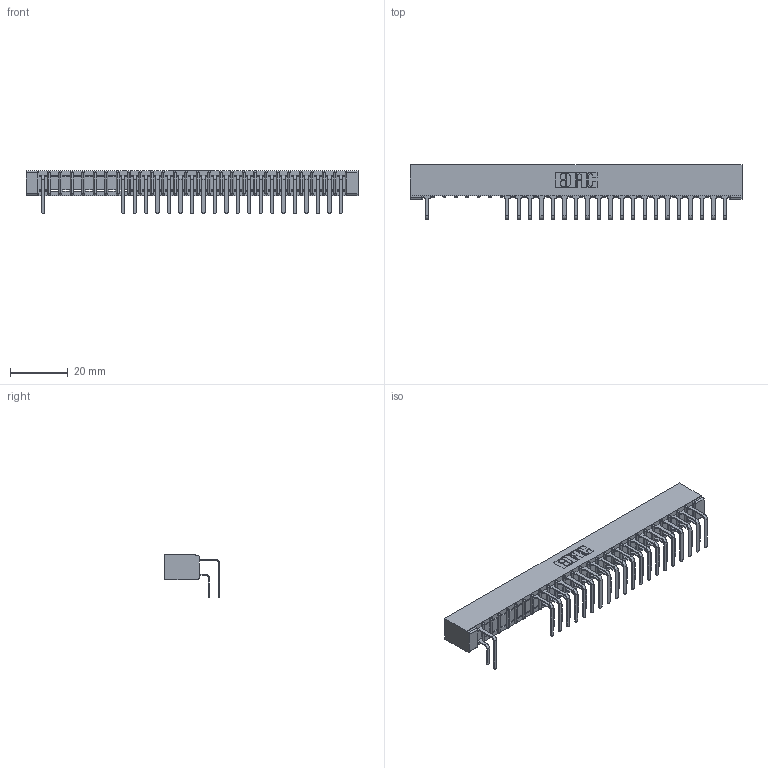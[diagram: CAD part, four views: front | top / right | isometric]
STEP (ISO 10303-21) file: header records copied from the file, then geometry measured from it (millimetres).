
FILE_DESCRIPTION (( 'STEP AP203' ), '1' );
FILE_NAME ('357-027-558-101.STEP', '2018-08-09T04:35:23', ( '' ), ( '' ), 'SwSTEP 2.0', 'SolidWorks 2016', '' );
FILE_SCHEMA (( 'CONFIG_CONTROL_DESIGN' ));
Length unit declared in the file: inch
Products named in the file (4): 307-290-001_558 - 2 (Single); 357-027-558-101; 307 Part_No Mounting Lugs; 307-290-001_558 559 - 1 (Single)
Assembly tree (42 placements, depth 2):
  357-027-558-101
    307 Part_No Mounting Lugs
    307-290-001_558 559 - 1 (Single)  x20
    307-290-001_558 - 2 (Single)  x21
Bounding box: 114.86 x 18.96 x 14.81 mm (x, y, z)
Volume: 7760.7 mm3; surface area: 14477.8 mm2
Topology: 42 solids, 42 shells, 2318 faces, 6537 edges, 4226 vertices
Faces by surface type: plane 1497, cylinder 765, sphere 56
Entity records: 26613 total; most frequent: CARTESIAN_POINT 4412, ORIENTED_EDGE 4382, DIRECTION 4313, EDGE_CURVE 2191, LINE 1675, VECTOR 1675, VERTEX_POINT 1418, AXIS2_PLACEMENT_3D 1319
